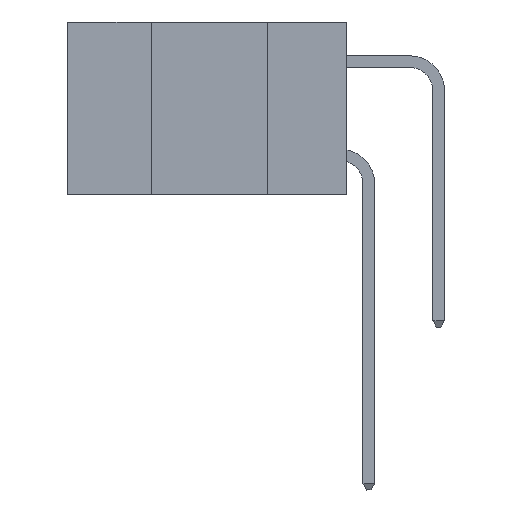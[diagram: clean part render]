
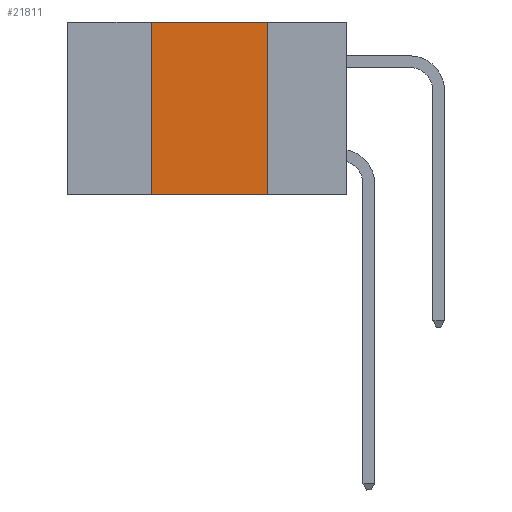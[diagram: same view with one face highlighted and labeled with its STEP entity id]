
A CAD part, left-side view. The second image highlights one B-rep face of the part: STEP entity #21811.
In plain terms, the highlighted planar face has unit normal (-1, 0, 0).
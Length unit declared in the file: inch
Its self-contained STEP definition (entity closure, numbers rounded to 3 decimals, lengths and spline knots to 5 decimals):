
#963 = LINE ( 'NONE', #12572, #16564 ) ;
#2284 = DIRECTION ( 'NONE',  ( 0., 0., -1. ) ) ;
#2573 = CARTESIAN_POINT ( 'NONE',  ( 0., 0.6, 0. ) ) ;
#3617 = VECTOR ( 'NONE', #28352, 39.37008 ) ;
#4267 = VERTEX_POINT ( 'NONE', #15565 ) ;
#4432 = EDGE_CURVE ( 'NONE', #28645, #25555, #27098, .T. ) ;
#4735 = EDGE_CURVE ( 'NONE', #11012, #25555, #963, .T. ) ;
#4815 = CARTESIAN_POINT ( 'NONE',  ( 0., 0.42, 0. ) ) ;
#6541 = CARTESIAN_POINT ( 'NONE',  ( 0., 0.42, -0.37 ) ) ;
#8646 = ORIENTED_EDGE ( 'NONE', *, *, #4432, .T. ) ;
#9251 = EDGE_CURVE ( 'NONE', #28645, #4267, #13304, .T. ) ;
#11012 = VERTEX_POINT ( 'NONE', #21285 ) ;
#11317 = DIRECTION ( 'NONE',  ( 0., -1., 0. ) ) ;
#12291 = DIRECTION ( 'NONE',  ( 0., 0., -1. ) ) ;
#12572 = CARTESIAN_POINT ( 'NONE',  ( 0., 0.17, 0. ) ) ;
#13074 = AXIS2_PLACEMENT_3D ( 'NONE', #2573, #15540, #2284 ) ;
#13155 = CARTESIAN_POINT ( 'NONE',  ( 0., 0.17, -0.37 ) ) ;
#13304 = LINE ( 'NONE', #4815, #16745 ) ;
#15122 = FACE_OUTER_BOUND ( 'NONE', #18819, .T. ) ;
#15540 = DIRECTION ( 'NONE',  ( 1., 0., 0. ) ) ;
#15565 = CARTESIAN_POINT ( 'NONE',  ( 0., 0.42, 0. ) ) ;
#15904 = VECTOR ( 'NONE', #11317, 39.37008 ) ;
#15930 = DIRECTION ( 'NONE',  ( 0., 0., 1. ) ) ;
#16564 = VECTOR ( 'NONE', #12291, 39.37008 ) ;
#16745 = VECTOR ( 'NONE', #15930, 39.37008 ) ;
#17839 = LINE ( 'NONE', #19675, #3617 ) ;
#18819 = EDGE_LOOP ( 'NONE', ( #18828, #27678, #19744, #8646 ) ) ;
#18828 = ORIENTED_EDGE ( 'NONE', *, *, #4735, .F. ) ;
#19675 = CARTESIAN_POINT ( 'NONE',  ( 0., 0.6, 0. ) ) ;
#19744 = ORIENTED_EDGE ( 'NONE', *, *, #9251, .F. ) ;
#20427 = CARTESIAN_POINT ( 'NONE',  ( 0., 0.6, -0.37 ) ) ;
#21235 = EDGE_CURVE ( 'NONE', #4267, #11012, #17839, .T. ) ;
#21285 = CARTESIAN_POINT ( 'NONE',  ( 0., 0.17, 0. ) ) ;
#21811 = ADVANCED_FACE ( 'NONE', ( #15122 ), #26775, .F. ) ;
#25555 = VERTEX_POINT ( 'NONE', #13155 ) ;
#26775 = PLANE ( 'NONE',  #13074 ) ;
#27098 = LINE ( 'NONE', #20427, #15904 ) ;
#27678 = ORIENTED_EDGE ( 'NONE', *, *, #21235, .F. ) ;
#28352 = DIRECTION ( 'NONE',  ( 0., -1., 0. ) ) ;
#28645 = VERTEX_POINT ( 'NONE', #6541 ) ;
